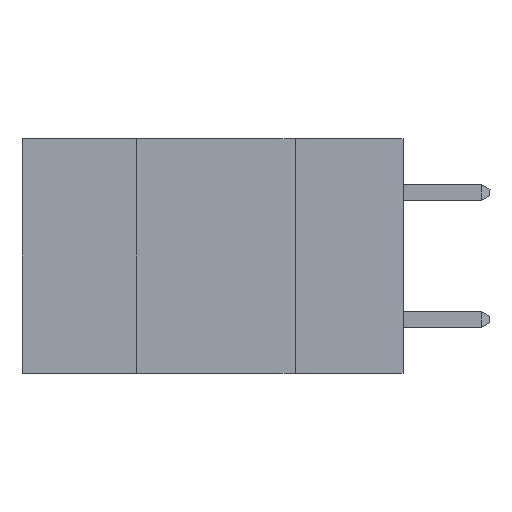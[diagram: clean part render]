
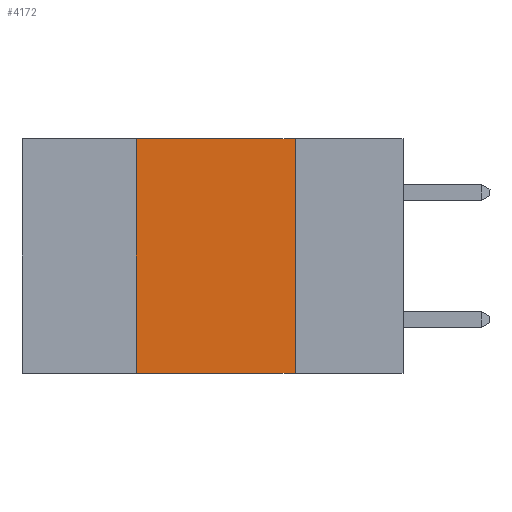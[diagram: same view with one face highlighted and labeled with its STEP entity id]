
A CAD part, left-side view. The second image highlights one B-rep face of the part: STEP entity #4172.
In plain terms, the highlighted planar face has unit normal (-1, 0, 0).
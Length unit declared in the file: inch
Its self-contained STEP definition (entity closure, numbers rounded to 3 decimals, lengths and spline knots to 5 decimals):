
#45 = PLANE ( 'NONE',  #4571 ) ;
#178 = ORIENTED_EDGE ( 'NONE', *, *, #11468, .T. ) ;
#325 = CARTESIAN_POINT ( 'NONE',  ( 0., 0.17, 0. ) ) ;
#808 = CARTESIAN_POINT ( 'NONE',  ( 0., 0.17, 0. ) ) ;
#1032 = DIRECTION ( 'NONE',  ( 0., 0., -1. ) ) ;
#1156 = VERTEX_POINT ( 'NONE', #808 ) ;
#1493 = CARTESIAN_POINT ( 'NONE',  ( 0., 0.17, -0.37 ) ) ;
#1619 = DIRECTION ( 'NONE',  ( 0., -1., 0. ) ) ;
#2500 = VECTOR ( 'NONE', #7525, 39.37008 ) ;
#2551 = VECTOR ( 'NONE', #1619, 39.37008 ) ;
#2745 = EDGE_CURVE ( 'NONE', #4809, #1156, #2829, .T. ) ;
#2829 = LINE ( 'NONE', #6962, #2551 ) ;
#4172 = ADVANCED_FACE ( 'NONE', ( #5872 ), #45, .F. ) ;
#4571 = AXIS2_PLACEMENT_3D ( 'NONE', #8974, #6428, #1032 ) ;
#4674 = ORIENTED_EDGE ( 'NONE', *, *, #10611, .F. ) ;
#4809 = VERTEX_POINT ( 'NONE', #10681 ) ;
#4898 = LINE ( 'NONE', #325, #2500 ) ;
#4944 = DIRECTION ( 'NONE',  ( 0., 0., 1. ) ) ;
#4961 = ORIENTED_EDGE ( 'NONE', *, *, #2745, .F. ) ;
#5225 = EDGE_LOOP ( 'NONE', ( #10421, #4961, #4674, #178 ) ) ;
#5823 = VERTEX_POINT ( 'NONE', #7652 ) ;
#5872 = FACE_OUTER_BOUND ( 'NONE', #5225, .T. ) ;
#6428 = DIRECTION ( 'NONE',  ( 1., 0., 0. ) ) ;
#6657 = CARTESIAN_POINT ( 'NONE',  ( 0., 0.42, 0. ) ) ;
#6962 = CARTESIAN_POINT ( 'NONE',  ( 0., 0.6, 0. ) ) ;
#7030 = LINE ( 'NONE', #6657, #9333 ) ;
#7525 = DIRECTION ( 'NONE',  ( 0., 0., -1. ) ) ;
#7652 = CARTESIAN_POINT ( 'NONE',  ( 0., 0.42, -0.37 ) ) ;
#7687 = VERTEX_POINT ( 'NONE', #1493 ) ;
#7798 = DIRECTION ( 'NONE',  ( 0., -1., 0. ) ) ;
#7830 = LINE ( 'NONE', #8670, #9864 ) ;
#8670 = CARTESIAN_POINT ( 'NONE',  ( 0., 0.6, -0.37 ) ) ;
#8974 = CARTESIAN_POINT ( 'NONE',  ( 0., 0.6, 0. ) ) ;
#9333 = VECTOR ( 'NONE', #4944, 39.37008 ) ;
#9440 = EDGE_CURVE ( 'NONE', #1156, #7687, #4898, .T. ) ;
#9864 = VECTOR ( 'NONE', #7798, 39.37008 ) ;
#10421 = ORIENTED_EDGE ( 'NONE', *, *, #9440, .F. ) ;
#10611 = EDGE_CURVE ( 'NONE', #5823, #4809, #7030, .T. ) ;
#10681 = CARTESIAN_POINT ( 'NONE',  ( 0., 0.42, 0. ) ) ;
#11468 = EDGE_CURVE ( 'NONE', #5823, #7687, #7830, .T. ) ;
